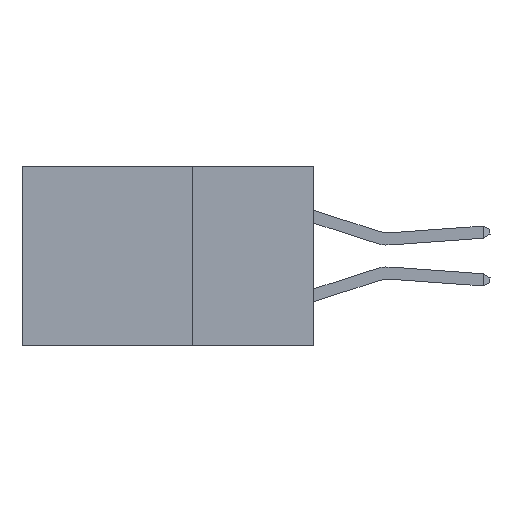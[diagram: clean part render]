
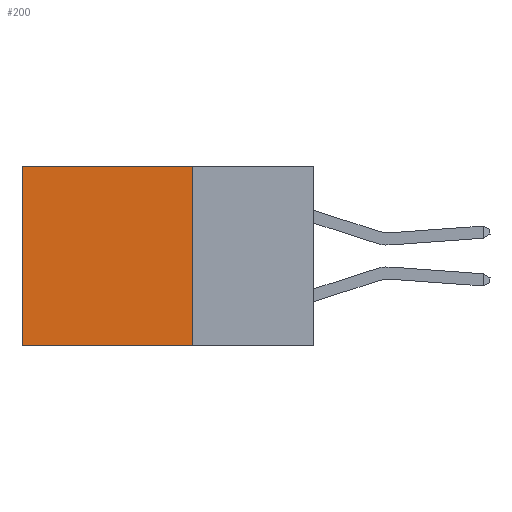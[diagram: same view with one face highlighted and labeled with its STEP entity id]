
A CAD part, left-side view. The second image highlights one B-rep face of the part: STEP entity #200.
In plain terms, the highlighted planar face has unit normal (-1, 0, 0).
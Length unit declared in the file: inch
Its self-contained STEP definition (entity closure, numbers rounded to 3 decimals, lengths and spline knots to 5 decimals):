
#200 = ADVANCED_FACE ( 'NONE', ( #9400 ), #17356, .F. ) ;
#528 = DIRECTION ( 'NONE',  ( 0., 0., -1. ) ) ;
#1063 = DIRECTION ( 'NONE',  ( 0., 0., -1. ) ) ;
#1886 = VECTOR ( 'NONE', #10521, 39.37008 ) ;
#2108 = VERTEX_POINT ( 'NONE', #3093 ) ;
#2193 = EDGE_LOOP ( 'NONE', ( #14067, #16516, #15004, #14128 ) ) ;
#2310 = CARTESIAN_POINT ( 'NONE',  ( 0.2875, 0.25, 0. ) ) ;
#3093 = CARTESIAN_POINT ( 'NONE',  ( 0.2875, 0.6, 0. ) ) ;
#5767 = CARTESIAN_POINT ( 'NONE',  ( 0.2875, 0.25, 0. ) ) ;
#7752 = DIRECTION ( 'NONE',  ( 1., 0., 0. ) ) ;
#8416 = CARTESIAN_POINT ( 'NONE',  ( 0.2875, 0.6, -0.37 ) ) ;
#8475 = AXIS2_PLACEMENT_3D ( 'NONE', #5767, #7752, #1063 ) ;
#8619 = LINE ( 'NONE', #13601, #1886 ) ;
#9400 = FACE_OUTER_BOUND ( 'NONE', #2193, .T. ) ;
#10096 = VERTEX_POINT ( 'NONE', #18452 ) ;
#10105 = CARTESIAN_POINT ( 'NONE',  ( 0.2875, 0.25, 0. ) ) ;
#10521 = DIRECTION ( 'NONE',  ( 0., 1., 0. ) ) ;
#11418 = VECTOR ( 'NONE', #528, 39.37008 ) ;
#11902 = LINE ( 'NONE', #12317, #15236 ) ;
#12317 = CARTESIAN_POINT ( 'NONE',  ( 0.2875, 0.6, 0. ) ) ;
#12430 = VERTEX_POINT ( 'NONE', #20987 ) ;
#13601 = CARTESIAN_POINT ( 'NONE',  ( 0.2875, 0.25, -0.37 ) ) ;
#14067 = ORIENTED_EDGE ( 'NONE', *, *, #17756, .T. ) ;
#14128 = ORIENTED_EDGE ( 'NONE', *, *, #15230, .T. ) ;
#14456 = EDGE_CURVE ( 'NONE', #12430, #10096, #17584, .T. ) ;
#15004 = ORIENTED_EDGE ( 'NONE', *, *, #14456, .F. ) ;
#15230 = EDGE_CURVE ( 'NONE', #12430, #2108, #18461, .T. ) ;
#15236 = VECTOR ( 'NONE', #16922, 39.37008 ) ;
#15928 = DIRECTION ( 'NONE',  ( 0., 1., 0. ) ) ;
#16301 = EDGE_CURVE ( 'NONE', #10096, #18823, #8619, .T. ) ;
#16516 = ORIENTED_EDGE ( 'NONE', *, *, #16301, .F. ) ;
#16922 = DIRECTION ( 'NONE',  ( 0., 0., -1. ) ) ;
#17356 = PLANE ( 'NONE',  #8475 ) ;
#17584 = LINE ( 'NONE', #10105, #11418 ) ;
#17756 = EDGE_CURVE ( 'NONE', #2108, #18823, #11902, .T. ) ;
#17941 = VECTOR ( 'NONE', #15928, 39.37008 ) ;
#18452 = CARTESIAN_POINT ( 'NONE',  ( 0.2875, 0.25, -0.37 ) ) ;
#18461 = LINE ( 'NONE', #2310, #17941 ) ;
#18823 = VERTEX_POINT ( 'NONE', #8416 ) ;
#20987 = CARTESIAN_POINT ( 'NONE',  ( 0.2875, 0.25, 0. ) ) ;
